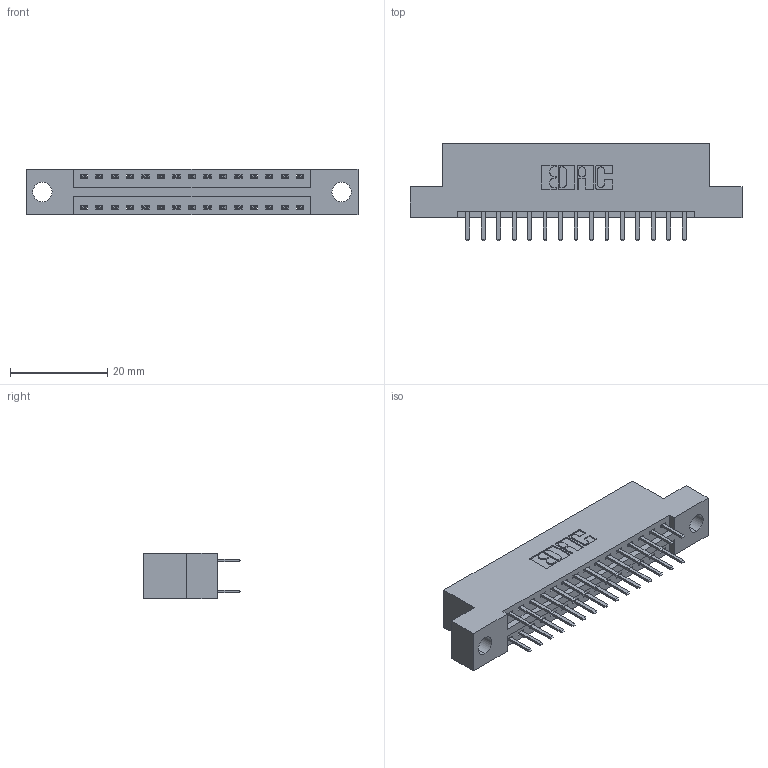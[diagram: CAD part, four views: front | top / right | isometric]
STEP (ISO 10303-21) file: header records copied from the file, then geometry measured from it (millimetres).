
FILE_DESCRIPTION (( 'STEP AP203' ), '1' );
FILE_NAME ('346-030-520-204.STEP', '2022-05-19T15:59:44', ( '' ), ( '' ), 'SwSTEP 2.0', 'SolidWorks 2020', '' );
FILE_SCHEMA (( 'CONFIG_CONTROL_DESIGN' ));
Length unit declared in the file: inch
Products named in the file (3): 345-292-001_345-293-120; 346-030-520-204; 346 Part_Flush Mounting Lugs - 0.156 Dia-TH
Assembly tree (31 placements, depth 2):
  346-030-520-204
    346 Part_Flush Mounting Lugs - 0.156 Dia-TH
    345-292-001_345-293-120  x30
Bounding box: 68.2 x 20.02 x 9.4 mm (x, y, z)
Volume: 6321.4 mm3; surface area: 8081.8 mm2
Topology: 31 solids, 31 shells, 1816 faces, 5255 edges, 3422 vertices
Faces by surface type: plane 1200, cylinder 616
Entity records: 13957 total; most frequent: CARTESIAN_POINT 2354, ORIENTED_EDGE 2274, DIRECTION 2113, EDGE_CURVE 1137, LINE 941, VECTOR 941, VERTEX_POINT 754, AXIS2_PLACEMENT_3D 586
